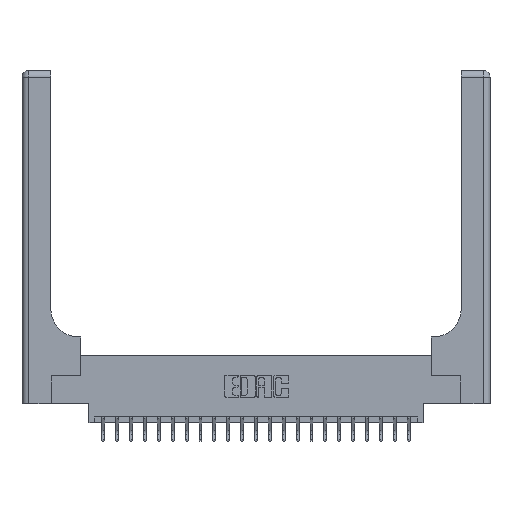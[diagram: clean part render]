
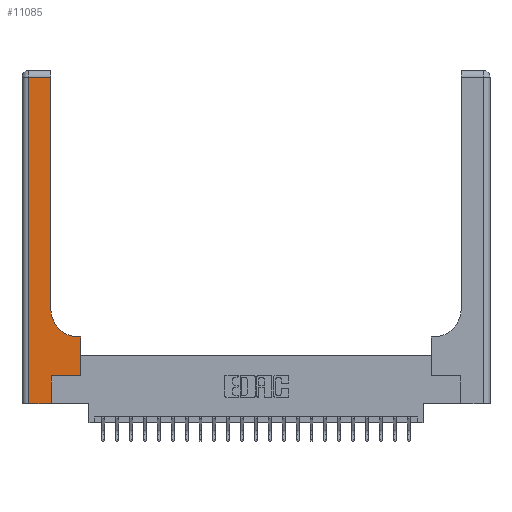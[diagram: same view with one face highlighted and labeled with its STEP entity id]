
A CAD part, top view. The second image highlights one B-rep face of the part: STEP entity #11085.
In plain terms, the highlighted planar face has unit normal (0, 0, 1).
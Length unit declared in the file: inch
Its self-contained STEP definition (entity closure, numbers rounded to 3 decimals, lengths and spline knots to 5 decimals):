
#119 = EDGE_CURVE ( 'NONE', #9795, #10346, #3067, .T. ) ;
#172 = LINE ( 'NONE', #14391, #8531 ) ;
#282 = EDGE_CURVE ( 'NONE', #21174, #7598, #10937, .T. ) ;
#372 = AXIS2_PLACEMENT_3D ( 'NONE', #18245, #21457, #21585 ) ;
#713 = CARTESIAN_POINT ( 'NONE',  ( 0., 0., 0.37 ) ) ;
#974 = VECTOR ( 'NONE', #1034, 39.37008 ) ;
#1034 = DIRECTION ( 'NONE',  ( 0., 1., 0. ) ) ;
#1390 = LINE ( 'NONE', #15936, #974 ) ;
#2254 = VECTOR ( 'NONE', #5961, 39.37008 ) ;
#2279 = CARTESIAN_POINT ( 'NONE',  ( 0.06, 0., 0.37 ) ) ;
#2665 = CARTESIAN_POINT ( 'NONE',  ( 0.26, 0.85, 0.37 ) ) ;
#3067 = LINE ( 'NONE', #713, #7296 ) ;
#3405 = DIRECTION ( 'NONE',  ( 0., 1., 0. ) ) ;
#3535 = DIRECTION ( 'NONE',  ( -1., 0., 0. ) ) ;
#3778 = EDGE_CURVE ( 'NONE', #9490, #15112, #1390, .T. ) ;
#3915 = EDGE_CURVE ( 'NONE', #19458, #12072, #11462, .T. ) ;
#4173 = LINE ( 'NONE', #7862, #2254 ) ;
#4610 = EDGE_CURVE ( 'NONE', #12072, #21174, #172, .T. ) ;
#5168 = CARTESIAN_POINT ( 'NONE',  ( 0.265, 0.25, 0.37 ) ) ;
#5712 = CARTESIAN_POINT ( 'NONE',  ( 0.265, 0., 0.37 ) ) ;
#5849 = CARTESIAN_POINT ( 'NONE',  ( 0.265, 0.25, 0.37 ) ) ;
#5893 = CARTESIAN_POINT ( 'NONE',  ( 0.528, 0.6, 0.37 ) ) ;
#5961 = DIRECTION ( 'NONE',  ( 0., -1., 0. ) ) ;
#6323 = VECTOR ( 'NONE', #9328, 39.37008 ) ;
#6536 = EDGE_CURVE ( 'NONE', #7598, #9490, #10674, .T. ) ;
#6945 = CARTESIAN_POINT ( 'NONE',  ( 0.51, 0.6, 0.37 ) ) ;
#7233 = CARTESIAN_POINT ( 'NONE',  ( 0.26, 0.6, 0.37 ) ) ;
#7296 = VECTOR ( 'NONE', #7859, 39.37008 ) ;
#7393 = ORIENTED_EDGE ( 'NONE', *, *, #16901, .T. ) ;
#7598 = VERTEX_POINT ( 'NONE', #6945 ) ;
#7859 = DIRECTION ( 'NONE',  ( 1., 0., 0. ) ) ;
#7862 = CARTESIAN_POINT ( 'NONE',  ( 0.06, 3., 0.37 ) ) ;
#8059 = EDGE_CURVE ( 'NONE', #15112, #11834, #21035, .T. ) ;
#8087 = LINE ( 'NONE', #21205, #9669 ) ;
#8531 = VECTOR ( 'NONE', #3405, 39.37008 ) ;
#9097 = DIRECTION ( 'NONE',  ( -1., 0., 0. ) ) ;
#9155 = EDGE_LOOP ( 'NONE', ( #18105, #11136, #7393, #18220, #11709, #22139, #18995, #17111, #16997 ) ) ;
#9328 = DIRECTION ( 'NONE',  ( 1., 0., 0. ) ) ;
#9490 = VERTEX_POINT ( 'NONE', #2665 ) ;
#9669 = VECTOR ( 'NONE', #15373, 39.37008 ) ;
#9795 = VERTEX_POINT ( 'NONE', #2279 ) ;
#10329 = DIRECTION ( 'NONE',  ( -1., 0., 0. ) ) ;
#10346 = VERTEX_POINT ( 'NONE', #5712 ) ;
#10674 = CIRCLE ( 'NONE', #372, 0.25 ) ;
#10755 = CARTESIAN_POINT ( 'NONE',  ( 0.528, 0.25, 0.37 ) ) ;
#10775 = CARTESIAN_POINT ( 'NONE',  ( 0., 3., 0.37 ) ) ;
#10937 = LINE ( 'NONE', #7233, #17591 ) ;
#11085 = ADVANCED_FACE ( 'NONE', ( #21841 ), #18279, .F. ) ;
#11136 = ORIENTED_EDGE ( 'NONE', *, *, #8059, .T. ) ;
#11462 = LINE ( 'NONE', #5849, #6323 ) ;
#11709 = ORIENTED_EDGE ( 'NONE', *, *, #21027, .T. ) ;
#11834 = VERTEX_POINT ( 'NONE', #19223 ) ;
#12072 = VERTEX_POINT ( 'NONE', #10755 ) ;
#14391 = CARTESIAN_POINT ( 'NONE',  ( 0.528, 0.25, 0.37 ) ) ;
#15112 = VERTEX_POINT ( 'NONE', #21217 ) ;
#15373 = DIRECTION ( 'NONE',  ( 0., 1., 0. ) ) ;
#15936 = CARTESIAN_POINT ( 'NONE',  ( 0.26, 3., 0.37 ) ) ;
#16384 = VECTOR ( 'NONE', #10329, 39.37008 ) ;
#16901 = EDGE_CURVE ( 'NONE', #11834, #9795, #4173, .T. ) ;
#16997 = ORIENTED_EDGE ( 'NONE', *, *, #6536, .T. ) ;
#17111 = ORIENTED_EDGE ( 'NONE', *, *, #282, .T. ) ;
#17591 = VECTOR ( 'NONE', #3535, 39.37008 ) ;
#17719 = CARTESIAN_POINT ( 'NONE',  ( 0., 2.94, 0.37 ) ) ;
#18040 = DIRECTION ( 'NONE',  ( 0., 0., -1. ) ) ;
#18071 = AXIS2_PLACEMENT_3D ( 'NONE', #10775, #18040, #9097 ) ;
#18105 = ORIENTED_EDGE ( 'NONE', *, *, #3778, .T. ) ;
#18220 = ORIENTED_EDGE ( 'NONE', *, *, #119, .T. ) ;
#18245 = CARTESIAN_POINT ( 'NONE',  ( 0.51, 0.85, 0.37 ) ) ;
#18279 = PLANE ( 'NONE',  #18071 ) ;
#18995 = ORIENTED_EDGE ( 'NONE', *, *, #4610, .T. ) ;
#19223 = CARTESIAN_POINT ( 'NONE',  ( 0.06, 2.94, 0.37 ) ) ;
#19458 = VERTEX_POINT ( 'NONE', #5168 ) ;
#21027 = EDGE_CURVE ( 'NONE', #10346, #19458, #8087, .T. ) ;
#21035 = LINE ( 'NONE', #17719, #16384 ) ;
#21174 = VERTEX_POINT ( 'NONE', #5893 ) ;
#21205 = CARTESIAN_POINT ( 'NONE',  ( 0.265, 0., 0.37 ) ) ;
#21217 = CARTESIAN_POINT ( 'NONE',  ( 0.26, 2.94, 0.37 ) ) ;
#21457 = DIRECTION ( 'NONE',  ( 0., 0., -1. ) ) ;
#21585 = DIRECTION ( 'NONE',  ( 1., 0., 0. ) ) ;
#21841 = FACE_OUTER_BOUND ( 'NONE', #9155, .T. ) ;
#22139 = ORIENTED_EDGE ( 'NONE', *, *, #3915, .T. ) ;
